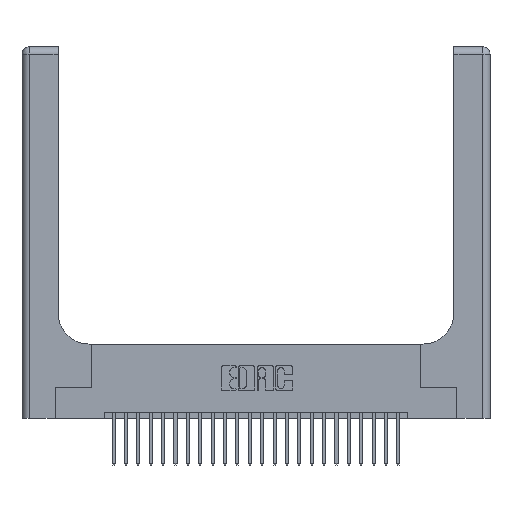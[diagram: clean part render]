
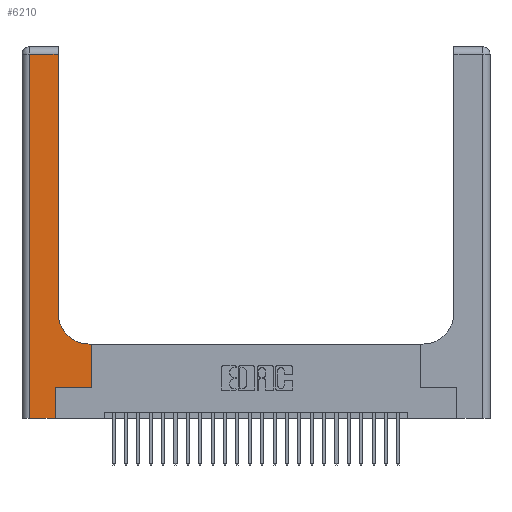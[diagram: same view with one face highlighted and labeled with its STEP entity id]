
A CAD part, top view. The second image highlights one B-rep face of the part: STEP entity #6210.
In plain terms, the highlighted planar face has unit normal (0, 0, 1).
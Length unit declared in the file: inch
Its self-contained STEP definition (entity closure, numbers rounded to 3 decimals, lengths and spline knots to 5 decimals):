
#828 = ORIENTED_EDGE ( 'NONE', *, *, #17702, .T. ) ;
#897 = CARTESIAN_POINT ( 'NONE',  ( 0., 2.94, 0.37 ) ) ;
#938 = LINE ( 'NONE', #22713, #21412 ) ;
#1013 = DIRECTION ( 'NONE',  ( -1., 0., 0. ) ) ;
#1263 = AXIS2_PLACEMENT_3D ( 'NONE', #3156, #9247, #1013 ) ;
#2085 = VECTOR ( 'NONE', #17485, 39.37008 ) ;
#2256 = ORIENTED_EDGE ( 'NONE', *, *, #11904, .T. ) ;
#2690 = VECTOR ( 'NONE', #7128, 39.37008 ) ;
#2715 = LINE ( 'NONE', #17207, #26079 ) ;
#3156 = CARTESIAN_POINT ( 'NONE',  ( 0., 3., 0.37 ) ) ;
#3426 = CARTESIAN_POINT ( 'NONE',  ( 0.269, 0., 0.37 ) ) ;
#5099 = CARTESIAN_POINT ( 'NONE',  ( 0.5585, 0.25, 0.37 ) ) ;
#5198 = DIRECTION ( 'NONE',  ( 1., 0., 0. ) ) ;
#6210 = ADVANCED_FACE ( 'NONE', ( #25140 ), #21667, .F. ) ;
#6843 = VERTEX_POINT ( 'NONE', #13017 ) ;
#6854 = LINE ( 'NONE', #23398, #2690 ) ;
#6893 = EDGE_CURVE ( 'NONE', #21676, #13261, #25112, .T. ) ;
#7128 = DIRECTION ( 'NONE',  ( 1., 0., 0. ) ) ;
#7197 = CARTESIAN_POINT ( 'NONE',  ( 0.2915, 3., 0.37 ) ) ;
#7423 = VERTEX_POINT ( 'NONE', #23796 ) ;
#7436 = EDGE_CURVE ( 'NONE', #16942, #19583, #26397, .T. ) ;
#7792 = CARTESIAN_POINT ( 'NONE',  ( 0.2915, 0.6, 0.37 ) ) ;
#7860 = EDGE_CURVE ( 'NONE', #19583, #21676, #21286, .T. ) ;
#8002 = LINE ( 'NONE', #5099, #24623 ) ;
#8877 = EDGE_CURVE ( 'NONE', #11594, #7423, #16430, .T. ) ;
#9247 = DIRECTION ( 'NONE',  ( 0., 0., -1. ) ) ;
#9635 = ORIENTED_EDGE ( 'NONE', *, *, #8877, .T. ) ;
#9824 = DIRECTION ( 'NONE',  ( -1., 0., 0. ) ) ;
#9935 = ORIENTED_EDGE ( 'NONE', *, *, #6893, .T. ) ;
#10445 = DIRECTION ( 'NONE',  ( 0., 1., 0. ) ) ;
#10800 = ORIENTED_EDGE ( 'NONE', *, *, #14192, .T. ) ;
#11235 = EDGE_CURVE ( 'NONE', #22852, #6843, #2715, .T. ) ;
#11594 = VERTEX_POINT ( 'NONE', #17075 ) ;
#11621 = CARTESIAN_POINT ( 'NONE',  ( 0.5415, 0.6, 0.37 ) ) ;
#11904 = EDGE_CURVE ( 'NONE', #6843, #13001, #6854, .T. ) ;
#12042 = CARTESIAN_POINT ( 'NONE',  ( 0.2915, 0.85, 0.37 ) ) ;
#13001 = VERTEX_POINT ( 'NONE', #3426 ) ;
#13017 = CARTESIAN_POINT ( 'NONE',  ( 0.06, 0., 0.37 ) ) ;
#13261 = VERTEX_POINT ( 'NONE', #19947 ) ;
#13474 = ORIENTED_EDGE ( 'NONE', *, *, #11235, .T. ) ;
#13537 = ORIENTED_EDGE ( 'NONE', *, *, #7436, .T. ) ;
#13639 = DIRECTION ( 'NONE',  ( 0., 1., 0. ) ) ;
#13670 = CARTESIAN_POINT ( 'NONE',  ( 0.269, 0.25, 0.37 ) ) ;
#13961 = ORIENTED_EDGE ( 'NONE', *, *, #7860, .T. ) ;
#14192 = EDGE_CURVE ( 'NONE', #13001, #11594, #938, .T. ) ;
#14633 = AXIS2_PLACEMENT_3D ( 'NONE', #21838, #16747, #5198 ) ;
#15329 = DIRECTION ( 'NONE',  ( 0., -1., 0. ) ) ;
#16015 = CARTESIAN_POINT ( 'NONE',  ( 0.06, 2.94, 0.37 ) ) ;
#16430 = LINE ( 'NONE', #13670, #21541 ) ;
#16434 = DIRECTION ( 'NONE',  ( 1., 0., 0. ) ) ;
#16747 = DIRECTION ( 'NONE',  ( 0., 0., -1. ) ) ;
#16942 = VERTEX_POINT ( 'NONE', #17242 ) ;
#17075 = CARTESIAN_POINT ( 'NONE',  ( 0.269, 0.25, 0.37 ) ) ;
#17091 = DIRECTION ( 'NONE',  ( -1., 0., 0. ) ) ;
#17207 = CARTESIAN_POINT ( 'NONE',  ( 0.06, 3., 0.37 ) ) ;
#17242 = CARTESIAN_POINT ( 'NONE',  ( 0.5585, 0.6, 0.37 ) ) ;
#17485 = DIRECTION ( 'NONE',  ( 0., 1., 0. ) ) ;
#17702 = EDGE_CURVE ( 'NONE', #7423, #16942, #8002, .T. ) ;
#18014 = EDGE_LOOP ( 'NONE', ( #9935, #19061, #13474, #2256, #10800, #9635, #828, #13537, #13961 ) ) ;
#19061 = ORIENTED_EDGE ( 'NONE', *, *, #21292, .T. ) ;
#19583 = VERTEX_POINT ( 'NONE', #11621 ) ;
#19947 = CARTESIAN_POINT ( 'NONE',  ( 0.2915, 2.94, 0.37 ) ) ;
#21286 = CIRCLE ( 'NONE', #14633, 0.25 ) ;
#21292 = EDGE_CURVE ( 'NONE', #13261, #22852, #25082, .T. ) ;
#21412 = VECTOR ( 'NONE', #13639, 39.37008 ) ;
#21541 = VECTOR ( 'NONE', #16434, 39.37008 ) ;
#21667 = PLANE ( 'NONE',  #1263 ) ;
#21676 = VERTEX_POINT ( 'NONE', #12042 ) ;
#21838 = CARTESIAN_POINT ( 'NONE',  ( 0.5415, 0.85, 0.37 ) ) ;
#22713 = CARTESIAN_POINT ( 'NONE',  ( 0.269, 0., 0.37 ) ) ;
#22852 = VERTEX_POINT ( 'NONE', #16015 ) ;
#23250 = VECTOR ( 'NONE', #9824, 39.37008 ) ;
#23398 = CARTESIAN_POINT ( 'NONE',  ( 0., 0., 0.37 ) ) ;
#23796 = CARTESIAN_POINT ( 'NONE',  ( 0.5585, 0.25, 0.37 ) ) ;
#24122 = VECTOR ( 'NONE', #17091, 39.37008 ) ;
#24623 = VECTOR ( 'NONE', #10445, 39.37008 ) ;
#25082 = LINE ( 'NONE', #897, #24122 ) ;
#25112 = LINE ( 'NONE', #7197, #2085 ) ;
#25140 = FACE_OUTER_BOUND ( 'NONE', #18014, .T. ) ;
#26079 = VECTOR ( 'NONE', #15329, 39.37008 ) ;
#26397 = LINE ( 'NONE', #7792, #23250 ) ;
